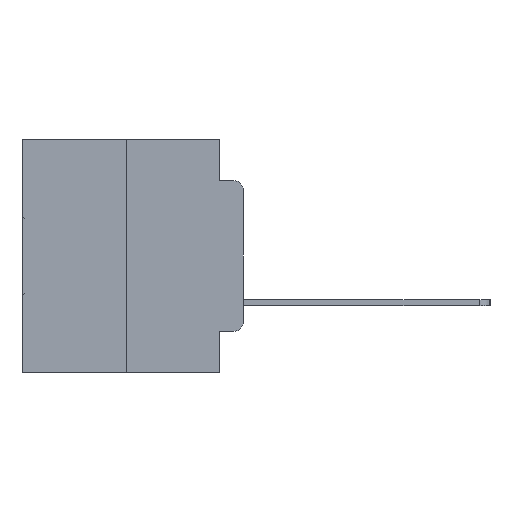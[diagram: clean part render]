
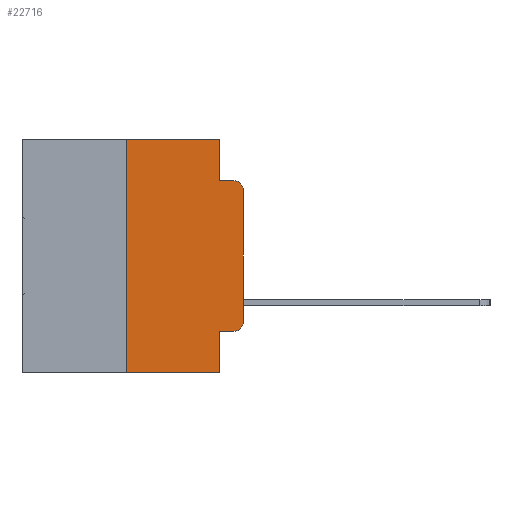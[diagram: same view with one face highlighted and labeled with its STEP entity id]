
A CAD part, left-side view. The second image highlights one B-rep face of the part: STEP entity #22716.
In plain terms, the highlighted planar face has unit normal (-1, 0, 0).
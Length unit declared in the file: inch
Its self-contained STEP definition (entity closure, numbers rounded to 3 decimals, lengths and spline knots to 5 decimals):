
#393 = CARTESIAN_POINT ( 'NONE',  ( 0., 0.02, -0.4115 ) ) ;
#1578 = CARTESIAN_POINT ( 'NONE',  ( 0., 0., -0.1085 ) ) ;
#2797 = ORIENTED_EDGE ( 'NONE', *, *, #23013, .F. ) ;
#2992 = ORIENTED_EDGE ( 'NONE', *, *, #19515, .T. ) ;
#3137 = CARTESIAN_POINT ( 'NONE',  ( 0., 0., 0. ) ) ;
#3757 = CARTESIAN_POINT ( 'NONE',  ( 0., 0.25, 0. ) ) ;
#3762 = DIRECTION ( 'NONE',  ( 0., -1., 0. ) ) ;
#3954 = VECTOR ( 'NONE', #20641, 39.37008 ) ;
#4504 = VERTEX_POINT ( 'NONE', #6511 ) ;
#4512 = ORIENTED_EDGE ( 'NONE', *, *, #22659, .F. ) ;
#4725 = LINE ( 'NONE', #13407, #22381 ) ;
#4887 = EDGE_CURVE ( 'NONE', #8982, #10366, #10489, .T. ) ;
#5010 = VECTOR ( 'NONE', #17115, 39.37008 ) ;
#6511 = CARTESIAN_POINT ( 'NONE',  ( 0., 0.02, -0.0885 ) ) ;
#7236 = LINE ( 'NONE', #26514, #24787 ) ;
#7273 = LINE ( 'NONE', #11856, #19351 ) ;
#7390 = CARTESIAN_POINT ( 'NONE',  ( 0., 0.02, -0.3915 ) ) ;
#7488 = CARTESIAN_POINT ( 'NONE',  ( 0., 0.473, 0. ) ) ;
#7592 = DIRECTION ( 'NONE',  ( 0., -1., 0. ) ) ;
#7979 = CARTESIAN_POINT ( 'NONE',  ( 0., 0.051, 0. ) ) ;
#8683 = DIRECTION ( 'NONE',  ( 1., 0., 0. ) ) ;
#8982 = VERTEX_POINT ( 'NONE', #25163 ) ;
#9169 = ORIENTED_EDGE ( 'NONE', *, *, #16244, .T. ) ;
#9311 = VECTOR ( 'NONE', #20013, 39.37008 ) ;
#9851 = DIRECTION ( 'NONE',  ( 0., 0., -1. ) ) ;
#10106 = AXIS2_PLACEMENT_3D ( 'NONE', #13721, #30064, #16146 ) ;
#10366 = VERTEX_POINT ( 'NONE', #16581 ) ;
#10489 = LINE ( 'NONE', #16434, #22444 ) ;
#11012 = ORIENTED_EDGE ( 'NONE', *, *, #28832, .T. ) ;
#11856 = CARTESIAN_POINT ( 'NONE',  ( 0., 0.051, 0. ) ) ;
#12268 = VERTEX_POINT ( 'NONE', #29838 ) ;
#12606 = DIRECTION ( 'NONE',  ( 0., 0., -1. ) ) ;
#13407 = CARTESIAN_POINT ( 'NONE',  ( 0., 0.473, -0.5 ) ) ;
#13721 = CARTESIAN_POINT ( 'NONE',  ( 0., 0.02, -0.1085 ) ) ;
#13780 = AXIS2_PLACEMENT_3D ( 'NONE', #20671, #8683, #25324 ) ;
#14471 = EDGE_LOOP ( 'NONE', ( #2992, #20331, #4512, #29357, #2797, #25521, #20614, #27486, #11012, #9169 ) ) ;
#14697 = EDGE_CURVE ( 'NONE', #26194, #4504, #18181, .T. ) ;
#15190 = AXIS2_PLACEMENT_3D ( 'NONE', #7390, #24118, #9851 ) ;
#15312 = VERTEX_POINT ( 'NONE', #23043 ) ;
#15641 = LINE ( 'NONE', #29606, #21233 ) ;
#15765 = DIRECTION ( 'NONE',  ( 0., -1., 0. ) ) ;
#16146 = DIRECTION ( 'NONE',  ( 0., 0., -1. ) ) ;
#16244 = EDGE_CURVE ( 'NONE', #24721, #17803, #24696, .T. ) ;
#16434 = CARTESIAN_POINT ( 'NONE',  ( 0., 0.051, 0. ) ) ;
#16581 = CARTESIAN_POINT ( 'NONE',  ( 0., 0.051, -0.5 ) ) ;
#17115 = DIRECTION ( 'NONE',  ( 0., -1., 0. ) ) ;
#17803 = VERTEX_POINT ( 'NONE', #20550 ) ;
#18181 = CIRCLE ( 'NONE', #10106, 0.02 ) ;
#19351 = VECTOR ( 'NONE', #26009, 39.37008 ) ;
#19515 = EDGE_CURVE ( 'NONE', #17803, #26194, #27454, .T. ) ;
#19687 = EDGE_CURVE ( 'NONE', #15312, #10366, #4725, .T. ) ;
#19912 = CARTESIAN_POINT ( 'NONE',  ( 0., 0.25, 0. ) ) ;
#20013 = DIRECTION ( 'NONE',  ( 0., 0., 1. ) ) ;
#20331 = ORIENTED_EDGE ( 'NONE', *, *, #14697, .T. ) ;
#20550 = CARTESIAN_POINT ( 'NONE',  ( 0., 0., -0.3915 ) ) ;
#20614 = ORIENTED_EDGE ( 'NONE', *, *, #19687, .T. ) ;
#20641 = DIRECTION ( 'NONE',  ( 0., 0., 1. ) ) ;
#20671 = CARTESIAN_POINT ( 'NONE',  ( 0., 0.473, 0. ) ) ;
#21095 = EDGE_CURVE ( 'NONE', #21898, #12268, #7273, .T. ) ;
#21233 = VECTOR ( 'NONE', #15765, 39.37008 ) ;
#21898 = VERTEX_POINT ( 'NONE', #7979 ) ;
#22375 = LINE ( 'NONE', #3757, #3954 ) ;
#22381 = VECTOR ( 'NONE', #3762, 39.37008 ) ;
#22444 = VECTOR ( 'NONE', #12606, 39.37008 ) ;
#22659 = EDGE_CURVE ( 'NONE', #12268, #4504, #15641, .T. ) ;
#22716 = ADVANCED_FACE ( 'NONE', ( #25931 ), #23010, .F. ) ;
#23010 = PLANE ( 'NONE',  #13780 ) ;
#23013 = EDGE_CURVE ( 'NONE', #26025, #21898, #30178, .T. ) ;
#23043 = CARTESIAN_POINT ( 'NONE',  ( 0., 0.25, -0.5 ) ) ;
#24118 = DIRECTION ( 'NONE',  ( -1., 0., 0. ) ) ;
#24696 = CIRCLE ( 'NONE', #15190, 0.02 ) ;
#24721 = VERTEX_POINT ( 'NONE', #393 ) ;
#24787 = VECTOR ( 'NONE', #7592, 39.37008 ) ;
#25163 = CARTESIAN_POINT ( 'NONE',  ( 0., 0.051, -0.4115 ) ) ;
#25324 = DIRECTION ( 'NONE',  ( 0., 0., -1. ) ) ;
#25521 = ORIENTED_EDGE ( 'NONE', *, *, #27301, .F. ) ;
#25931 = FACE_OUTER_BOUND ( 'NONE', #14471, .T. ) ;
#26009 = DIRECTION ( 'NONE',  ( 0., 0., -1. ) ) ;
#26025 = VERTEX_POINT ( 'NONE', #19912 ) ;
#26194 = VERTEX_POINT ( 'NONE', #1578 ) ;
#26514 = CARTESIAN_POINT ( 'NONE',  ( 0., 0.051, -0.4115 ) ) ;
#27301 = EDGE_CURVE ( 'NONE', #15312, #26025, #22375, .T. ) ;
#27454 = LINE ( 'NONE', #3137, #9311 ) ;
#27486 = ORIENTED_EDGE ( 'NONE', *, *, #4887, .F. ) ;
#28832 = EDGE_CURVE ( 'NONE', #8982, #24721, #7236, .T. ) ;
#29357 = ORIENTED_EDGE ( 'NONE', *, *, #21095, .F. ) ;
#29606 = CARTESIAN_POINT ( 'NONE',  ( 0., 0.051, -0.0885 ) ) ;
#29838 = CARTESIAN_POINT ( 'NONE',  ( 0., 0.051, -0.0885 ) ) ;
#30064 = DIRECTION ( 'NONE',  ( -1., 0., 0. ) ) ;
#30178 = LINE ( 'NONE', #7488, #5010 ) ;
